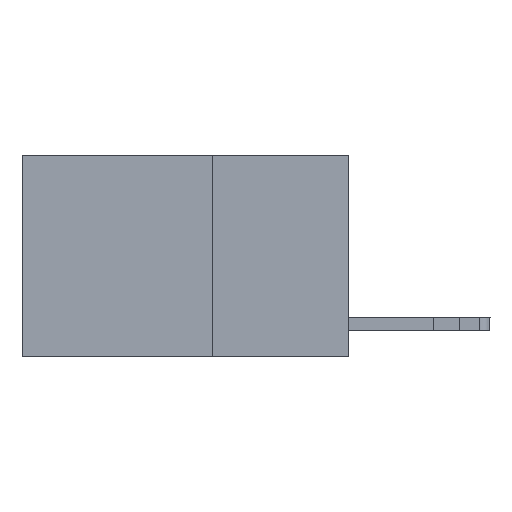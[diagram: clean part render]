
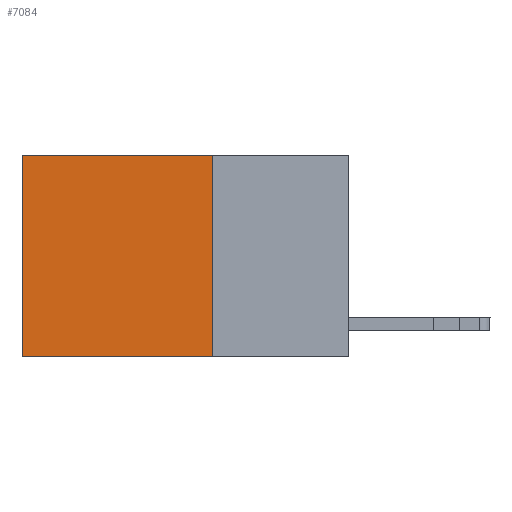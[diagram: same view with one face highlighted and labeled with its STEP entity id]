
A CAD part, left-side view. The second image highlights one B-rep face of the part: STEP entity #7084.
In plain terms, the highlighted planar face has unit normal (-1, 0, 0).
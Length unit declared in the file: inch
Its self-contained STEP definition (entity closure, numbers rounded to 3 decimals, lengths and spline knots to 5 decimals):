
#201 = VERTEX_POINT ( 'NONE', #12579 ) ;
#2180 = FACE_OUTER_BOUND ( 'NONE', #8961, .T. ) ;
#4853 = DIRECTION ( 'NONE',  ( 1., 0., 0. ) ) ;
#4989 = EDGE_CURVE ( 'NONE', #9591, #11357, #16264, .T. ) ;
#5139 = VECTOR ( 'NONE', #5209, 39.37008 ) ;
#5209 = DIRECTION ( 'NONE',  ( 0., 0., -1. ) ) ;
#5644 = CARTESIAN_POINT ( 'NONE',  ( 0.2625, 0.6, -0.37 ) ) ;
#6714 = AXIS2_PLACEMENT_3D ( 'NONE', #17257, #4853, #19334 ) ;
#7084 = ADVANCED_FACE ( 'NONE', ( #2180 ), #10669, .F. ) ;
#8346 = ORIENTED_EDGE ( 'NONE', *, *, #15053, .T. ) ;
#8606 = VECTOR ( 'NONE', #23306, 39.37008 ) ;
#8903 = DIRECTION ( 'NONE',  ( 0., 1., 0. ) ) ;
#8961 = EDGE_LOOP ( 'NONE', ( #17812, #17184, #12238, #8346 ) ) ;
#9591 = VERTEX_POINT ( 'NONE', #17862 ) ;
#10669 = PLANE ( 'NONE',  #6714 ) ;
#11357 = VERTEX_POINT ( 'NONE', #5644 ) ;
#12238 = ORIENTED_EDGE ( 'NONE', *, *, #14424, .F. ) ;
#12579 = CARTESIAN_POINT ( 'NONE',  ( 0.2625, 0.25, 0. ) ) ;
#13456 = CARTESIAN_POINT ( 'NONE',  ( 0.2625, 0.6, 0. ) ) ;
#13741 = VECTOR ( 'NONE', #8903, 39.37008 ) ;
#14121 = LINE ( 'NONE', #21282, #8606 ) ;
#14424 = EDGE_CURVE ( 'NONE', #201, #9591, #14121, .T. ) ;
#15053 = EDGE_CURVE ( 'NONE', #201, #16580, #19217, .T. ) ;
#16264 = LINE ( 'NONE', #23004, #20427 ) ;
#16478 = EDGE_CURVE ( 'NONE', #16580, #11357, #26367, .T. ) ;
#16580 = VERTEX_POINT ( 'NONE', #22058 ) ;
#17123 = CARTESIAN_POINT ( 'NONE',  ( 0.2625, 0.25, 0. ) ) ;
#17184 = ORIENTED_EDGE ( 'NONE', *, *, #4989, .F. ) ;
#17257 = CARTESIAN_POINT ( 'NONE',  ( 0.2625, 0.25, 0. ) ) ;
#17812 = ORIENTED_EDGE ( 'NONE', *, *, #16478, .T. ) ;
#17862 = CARTESIAN_POINT ( 'NONE',  ( 0.2625, 0.25, -0.37 ) ) ;
#19217 = LINE ( 'NONE', #17123, #13741 ) ;
#19334 = DIRECTION ( 'NONE',  ( 0., 0., -1. ) ) ;
#20427 = VECTOR ( 'NONE', #20990, 39.37008 ) ;
#20990 = DIRECTION ( 'NONE',  ( 0., 1., 0. ) ) ;
#21282 = CARTESIAN_POINT ( 'NONE',  ( 0.2625, 0.25, 0. ) ) ;
#22058 = CARTESIAN_POINT ( 'NONE',  ( 0.2625, 0.6, 0. ) ) ;
#23004 = CARTESIAN_POINT ( 'NONE',  ( 0.2625, 0.25, -0.37 ) ) ;
#23306 = DIRECTION ( 'NONE',  ( 0., 0., -1. ) ) ;
#26367 = LINE ( 'NONE', #13456, #5139 ) ;
